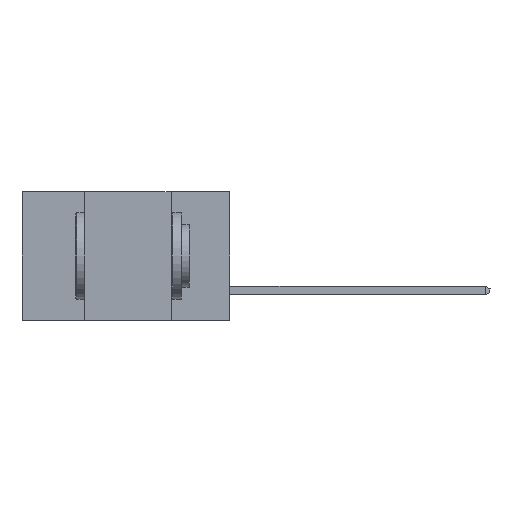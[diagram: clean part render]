
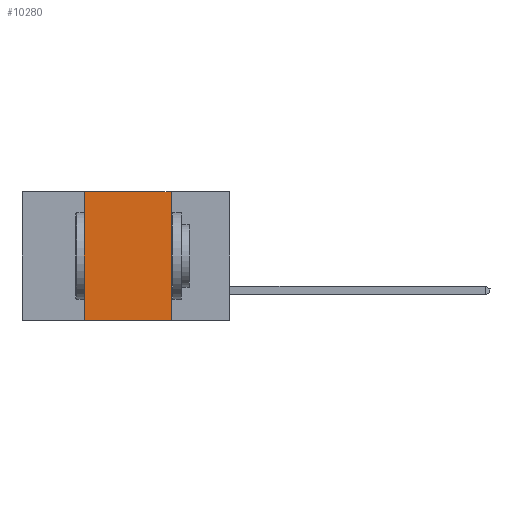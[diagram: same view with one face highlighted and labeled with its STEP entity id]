
A CAD part, left-side view. The second image highlights one B-rep face of the part: STEP entity #10280.
In plain terms, the highlighted planar face has unit normal (-1, 0, 0).
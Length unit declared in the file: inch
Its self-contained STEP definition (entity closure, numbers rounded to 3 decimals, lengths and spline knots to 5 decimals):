
#2 = LINE ( 'NONE', #3764, #3703 ) ;
#119 = ORIENTED_EDGE ( 'NONE', *, *, #752, .F. ) ;
#520 = CARTESIAN_POINT ( 'NONE',  ( 0., 0.17, -0.37 ) ) ;
#752 = EDGE_CURVE ( 'NONE', #9882, #6116, #3547, .T. ) ;
#835 = ORIENTED_EDGE ( 'NONE', *, *, #10035, .T. ) ;
#1164 = DIRECTION ( 'NONE',  ( 0., 0., -1. ) ) ;
#1231 = CARTESIAN_POINT ( 'NONE',  ( 0., 0.17, -0.37 ) ) ;
#1283 = CARTESIAN_POINT ( 'NONE',  ( 0., 0.17, 0. ) ) ;
#1531 = ORIENTED_EDGE ( 'NONE', *, *, #8942, .F. ) ;
#2043 = AXIS2_PLACEMENT_3D ( 'NONE', #5449, #4460, #6590 ) ;
#2945 = CARTESIAN_POINT ( 'NONE',  ( 0., 0.42, 0. ) ) ;
#3375 = PLANE ( 'NONE',  #2043 ) ;
#3450 = VERTEX_POINT ( 'NONE', #1283 ) ;
#3547 = LINE ( 'NONE', #8449, #6572 ) ;
#3703 = VECTOR ( 'NONE', #7886, 39.37008 ) ;
#3764 = CARTESIAN_POINT ( 'NONE',  ( 0., 0.6, -0.37 ) ) ;
#4460 = DIRECTION ( 'NONE',  ( 1., 0., 0. ) ) ;
#4586 = VECTOR ( 'NONE', #1164, 39.37008 ) ;
#4669 = CARTESIAN_POINT ( 'NONE',  ( 0., 0.42, -0.37 ) ) ;
#5449 = CARTESIAN_POINT ( 'NONE',  ( 0., 0.6, 0. ) ) ;
#5772 = ORIENTED_EDGE ( 'NONE', *, *, #5938, .F. ) ;
#5938 = EDGE_CURVE ( 'NONE', #3450, #10269, #8084, .T. ) ;
#5941 = VECTOR ( 'NONE', #12045, 39.37008 ) ;
#6116 = VERTEX_POINT ( 'NONE', #2945 ) ;
#6233 = EDGE_LOOP ( 'NONE', ( #5772, #1531, #119, #835 ) ) ;
#6332 = DIRECTION ( 'NONE',  ( 0., 0., 1. ) ) ;
#6572 = VECTOR ( 'NONE', #6332, 39.37008 ) ;
#6590 = DIRECTION ( 'NONE',  ( 0., 0., -1. ) ) ;
#7161 = CARTESIAN_POINT ( 'NONE',  ( 0., 0.6, 0. ) ) ;
#7886 = DIRECTION ( 'NONE',  ( 0., -1., 0. ) ) ;
#8078 = LINE ( 'NONE', #7161, #5941 ) ;
#8084 = LINE ( 'NONE', #1231, #4586 ) ;
#8449 = CARTESIAN_POINT ( 'NONE',  ( 0., 0.42, -0.37 ) ) ;
#8942 = EDGE_CURVE ( 'NONE', #6116, #3450, #8078, .T. ) ;
#9438 = FACE_OUTER_BOUND ( 'NONE', #6233, .T. ) ;
#9882 = VERTEX_POINT ( 'NONE', #4669 ) ;
#10035 = EDGE_CURVE ( 'NONE', #9882, #10269, #2, .T. ) ;
#10269 = VERTEX_POINT ( 'NONE', #520 ) ;
#10280 = ADVANCED_FACE ( 'NONE', ( #9438 ), #3375, .F. ) ;
#12045 = DIRECTION ( 'NONE',  ( 0., -1., 0. ) ) ;
